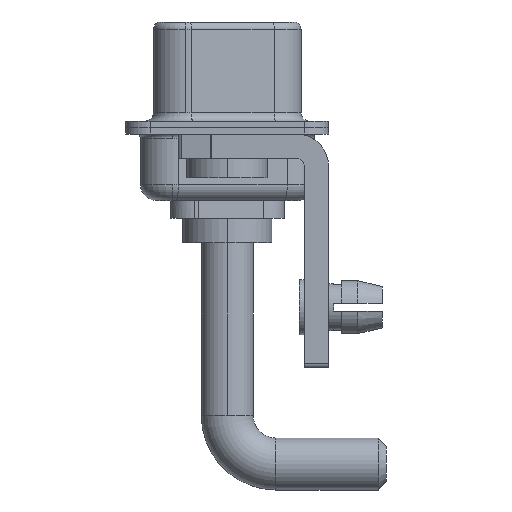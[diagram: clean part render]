
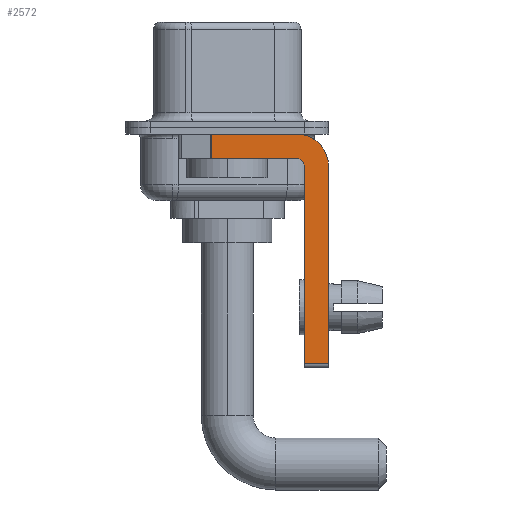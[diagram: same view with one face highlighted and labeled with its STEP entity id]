
A CAD part, left-side view. The second image highlights one B-rep face of the part: STEP entity #2572.
In plain terms, the highlighted planar face has unit normal (-1, 0, 0).
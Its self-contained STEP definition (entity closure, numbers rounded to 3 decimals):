
#112 = EDGE_CURVE ( 'NONE', #5637, #6201, #7438, .T. ) ;
#253 = CARTESIAN_POINT ( 'NONE',  ( -2.9, 3., -0.4 ) ) ;
#878 = LINE ( 'NONE', #2255, #3019 ) ;
#1104 = VERTEX_POINT ( 'NONE', #15278 ) ;
#1989 = EDGE_LOOP ( 'NONE', ( #5594, #14788, #12195, #7532, #11621, #6241, #12065, #14943 ) ) ;
#2061 = DIRECTION ( 'NONE',  ( 0., 0., -1. ) ) ;
#2255 = CARTESIAN_POINT ( 'NONE',  ( -2.9, 0.978, -1.9 ) ) ;
#2572 = ADVANCED_FACE ( 'NONE', ( #8857 ), #4933, .F. ) ;
#2645 = DIRECTION ( 'NONE',  ( 0., 0., -1. ) ) ;
#2893 = CIRCLE ( 'NONE', #11638, 2. ) ;
#3019 = VECTOR ( 'NONE', #11232, 1000. ) ;
#3244 = EDGE_CURVE ( 'NONE', #12102, #7267, #7099, .T. ) ;
#3907 = DIRECTION ( 'NONE',  ( 1., 0., 0. ) ) ;
#4114 = DIRECTION ( 'NONE',  ( 0., -1., 0. ) ) ;
#4466 = VECTOR ( 'NONE', #11340, 1000. ) ;
#4492 = DIRECTION ( 'NONE',  ( 0., 1., 0. ) ) ;
#4801 = EDGE_CURVE ( 'NONE', #11161, #10618, #13539, .T. ) ;
#4814 = CARTESIAN_POINT ( 'NONE',  ( -2.9, 0.978, -1.9 ) ) ;
#4933 = PLANE ( 'NONE',  #8165 ) ;
#5594 = ORIENTED_EDGE ( 'NONE', *, *, #3244, .F. ) ;
#5637 = VERTEX_POINT ( 'NONE', #14687 ) ;
#6135 = LINE ( 'NONE', #10253, #12402 ) ;
#6201 = VERTEX_POINT ( 'NONE', #15956 ) ;
#6241 = ORIENTED_EDGE ( 'NONE', *, *, #4801, .T. ) ;
#6463 = EDGE_CURVE ( 'NONE', #12102, #14081, #878, .T. ) ;
#7099 = LINE ( 'NONE', #253, #11446 ) ;
#7267 = VERTEX_POINT ( 'NONE', #15121 ) ;
#7438 = CIRCLE ( 'NONE', #10452, 0.5 ) ;
#7497 = CARTESIAN_POINT ( 'NONE',  ( -2.9, -4.25, -2.4 ) ) ;
#7522 = DIRECTION ( 'NONE',  ( 1., 0., 0. ) ) ;
#7532 = ORIENTED_EDGE ( 'NONE', *, *, #112, .F. ) ;
#8165 = AXIS2_PLACEMENT_3D ( 'NONE', #7497, #3907, #10157 ) ;
#8401 = DIRECTION ( 'NONE',  ( 0., 0., 1. ) ) ;
#8521 = CARTESIAN_POINT ( 'NONE',  ( -2.9, -4.25, -1.9 ) ) ;
#8760 = CARTESIAN_POINT ( 'NONE',  ( -2.9, -6.25, -14.55 ) ) ;
#8857 = FACE_OUTER_BOUND ( 'NONE', #1989, .T. ) ;
#9097 = EDGE_CURVE ( 'NONE', #6201, #14081, #13840, .T. ) ;
#10076 = EDGE_CURVE ( 'NONE', #1104, #10618, #6135, .T. ) ;
#10157 = DIRECTION ( 'NONE',  ( 0., 0., -1. ) ) ;
#10253 = CARTESIAN_POINT ( 'NONE',  ( -2.9, -6.25, -2.4 ) ) ;
#10452 = AXIS2_PLACEMENT_3D ( 'NONE', #12107, #10641, #8401 ) ;
#10581 = EDGE_CURVE ( 'NONE', #11161, #5637, #16838, .T. ) ;
#10618 = VERTEX_POINT ( 'NONE', #8760 ) ;
#10624 = CARTESIAN_POINT ( 'NONE',  ( -2.9, -4.25, -14.55 ) ) ;
#10641 = DIRECTION ( 'NONE',  ( -1., 0., 0. ) ) ;
#11161 = VERTEX_POINT ( 'NONE', #16648 ) ;
#11232 = DIRECTION ( 'NONE',  ( 0., 0., -1. ) ) ;
#11340 = DIRECTION ( 'NONE',  ( 0., 0., 1. ) ) ;
#11446 = VECTOR ( 'NONE', #13379, 1000. ) ;
#11621 = ORIENTED_EDGE ( 'NONE', *, *, #10581, .F. ) ;
#11638 = AXIS2_PLACEMENT_3D ( 'NONE', #16620, #7522, #2061 ) ;
#12014 = CARTESIAN_POINT ( 'NONE',  ( -2.9, 0.978, -0.4 ) ) ;
#12065 = ORIENTED_EDGE ( 'NONE', *, *, #10076, .F. ) ;
#12102 = VERTEX_POINT ( 'NONE', #12014 ) ;
#12107 = CARTESIAN_POINT ( 'NONE',  ( -2.9, -4.25, -2.4 ) ) ;
#12195 = ORIENTED_EDGE ( 'NONE', *, *, #9097, .F. ) ;
#12402 = VECTOR ( 'NONE', #2645, 1000. ) ;
#13379 = DIRECTION ( 'NONE',  ( 0., -1., 0. ) ) ;
#13539 = LINE ( 'NONE', #10624, #13906 ) ;
#13840 = LINE ( 'NONE', #8521, #16467 ) ;
#13906 = VECTOR ( 'NONE', #4114, 1000. ) ;
#14081 = VERTEX_POINT ( 'NONE', #4814 ) ;
#14348 = EDGE_CURVE ( 'NONE', #7267, #1104, #2893, .T. ) ;
#14687 = CARTESIAN_POINT ( 'NONE',  ( -2.9, -4.75, -2.4 ) ) ;
#14788 = ORIENTED_EDGE ( 'NONE', *, *, #6463, .T. ) ;
#14943 = ORIENTED_EDGE ( 'NONE', *, *, #14348, .F. ) ;
#15121 = CARTESIAN_POINT ( 'NONE',  ( -2.9, -4.25, -0.4 ) ) ;
#15278 = CARTESIAN_POINT ( 'NONE',  ( -2.9, -6.25, -2.4 ) ) ;
#15956 = CARTESIAN_POINT ( 'NONE',  ( -2.9, -4.25, -1.9 ) ) ;
#16467 = VECTOR ( 'NONE', #4492, 1000. ) ;
#16620 = CARTESIAN_POINT ( 'NONE',  ( -2.9, -4.25, -2.4 ) ) ;
#16648 = CARTESIAN_POINT ( 'NONE',  ( -2.9, -4.75, -14.55 ) ) ;
#16838 = LINE ( 'NONE', #16932, #4466 ) ;
#16932 = CARTESIAN_POINT ( 'NONE',  ( -2.9, -4.75, -14.8 ) ) ;
